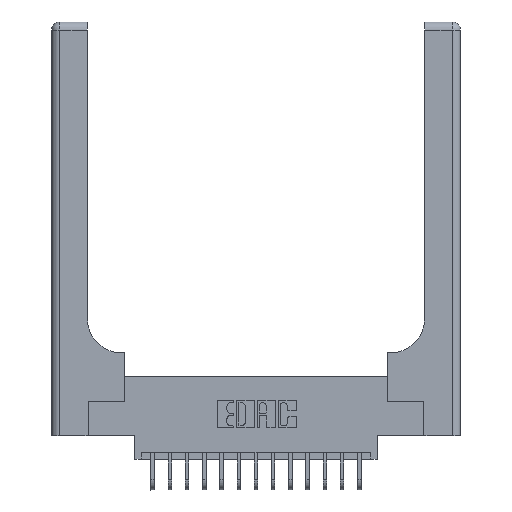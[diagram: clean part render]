
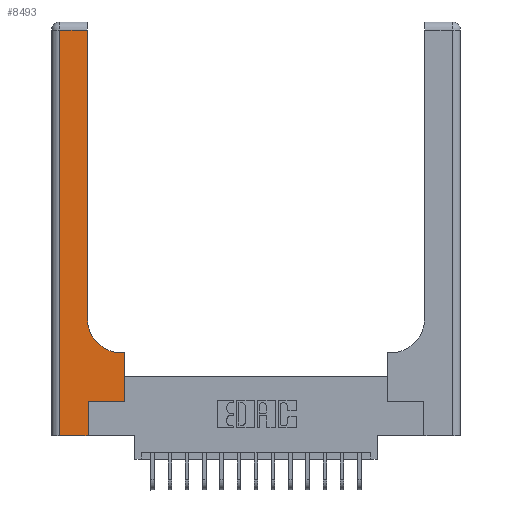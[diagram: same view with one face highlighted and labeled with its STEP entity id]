
A CAD part, top view. The second image highlights one B-rep face of the part: STEP entity #8493.
In plain terms, the highlighted planar face has unit normal (0, 0, 1).
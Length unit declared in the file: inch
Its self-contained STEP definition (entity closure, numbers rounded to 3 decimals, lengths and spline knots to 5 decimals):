
#258 = CARTESIAN_POINT ( 'NONE',  ( 0.26, 0.85, 0.37 ) ) ;
#544 = VERTEX_POINT ( 'NONE', #15797 ) ;
#574 = EDGE_CURVE ( 'NONE', #988, #16833, #8580, .T. ) ;
#685 = CARTESIAN_POINT ( 'NONE',  ( 0.265, 0., 0.37 ) ) ;
#988 = VERTEX_POINT ( 'NONE', #12697 ) ;
#1490 = DIRECTION ( 'NONE',  ( 0., 0., -1. ) ) ;
#1655 = FACE_OUTER_BOUND ( 'NONE', #15881, .T. ) ;
#2187 = VECTOR ( 'NONE', #7124, 39.37008 ) ;
#3043 = CARTESIAN_POINT ( 'NONE',  ( 0.528, 0.6, 0.37 ) ) ;
#3172 = EDGE_CURVE ( 'NONE', #544, #18215, #10111, .T. ) ;
#3312 = VECTOR ( 'NONE', #18444, 39.37008 ) ;
#3699 = DIRECTION ( 'NONE',  ( 0., 1., 0. ) ) ;
#4691 = ORIENTED_EDGE ( 'NONE', *, *, #3172, .T. ) ;
#5363 = EDGE_CURVE ( 'NONE', #16833, #6987, #13559, .T. ) ;
#5413 = VECTOR ( 'NONE', #5875, 39.37008 ) ;
#5875 = DIRECTION ( 'NONE',  ( -1., 0., 0. ) ) ;
#6525 = VERTEX_POINT ( 'NONE', #685 ) ;
#6743 = VECTOR ( 'NONE', #18944, 39.37008 ) ;
#6987 = VERTEX_POINT ( 'NONE', #11197 ) ;
#7124 = DIRECTION ( 'NONE',  ( 0., 1., 0. ) ) ;
#7527 = EDGE_CURVE ( 'NONE', #6525, #14617, #11607, .T. ) ;
#7754 = DIRECTION ( 'NONE',  ( 1., 0., 0. ) ) ;
#7800 = DIRECTION ( 'NONE',  ( -1., 0., 0. ) ) ;
#8045 = EDGE_CURVE ( 'NONE', #18215, #6525, #16307, .T. ) ;
#8174 = ORIENTED_EDGE ( 'NONE', *, *, #14600, .T. ) ;
#8195 = EDGE_CURVE ( 'NONE', #12801, #8676, #13699, .T. ) ;
#8493 = ADVANCED_FACE ( 'NONE', ( #1655 ), #19212, .F. ) ;
#8580 = LINE ( 'NONE', #11336, #2187 ) ;
#8676 = VERTEX_POINT ( 'NONE', #18752 ) ;
#8742 = AXIS2_PLACEMENT_3D ( 'NONE', #18163, #16744, #12337 ) ;
#8985 = CARTESIAN_POINT ( 'NONE',  ( 0., 0., 0.37 ) ) ;
#9067 = CARTESIAN_POINT ( 'NONE',  ( 0.26, 0.6, 0.37 ) ) ;
#9214 = EDGE_CURVE ( 'NONE', #8676, #544, #17437, .T. ) ;
#9702 = VECTOR ( 'NONE', #7754, 39.37008 ) ;
#10111 = LINE ( 'NONE', #10666, #10379 ) ;
#10379 = VECTOR ( 'NONE', #14846, 39.37008 ) ;
#10666 = CARTESIAN_POINT ( 'NONE',  ( 0.06, 3., 0.37 ) ) ;
#10813 = CARTESIAN_POINT ( 'NONE',  ( 0.26, 3., 0.37 ) ) ;
#10923 = VECTOR ( 'NONE', #3699, 39.37008 ) ;
#10976 = AXIS2_PLACEMENT_3D ( 'NONE', #13743, #1490, #7800 ) ;
#11197 = CARTESIAN_POINT ( 'NONE',  ( 0.51, 0.6, 0.37 ) ) ;
#11312 = EDGE_CURVE ( 'NONE', #6987, #12801, #18804, .T. ) ;
#11336 = CARTESIAN_POINT ( 'NONE',  ( 0.528, 0.25, 0.37 ) ) ;
#11607 = LINE ( 'NONE', #18727, #10923 ) ;
#12337 = DIRECTION ( 'NONE',  ( 1., 0., 0. ) ) ;
#12697 = CARTESIAN_POINT ( 'NONE',  ( 0.528, 0.25, 0.37 ) ) ;
#12801 = VERTEX_POINT ( 'NONE', #258 ) ;
#13238 = ORIENTED_EDGE ( 'NONE', *, *, #7527, .T. ) ;
#13462 = ORIENTED_EDGE ( 'NONE', *, *, #9214, .T. ) ;
#13559 = LINE ( 'NONE', #9067, #6743 ) ;
#13699 = LINE ( 'NONE', #10813, #3312 ) ;
#13743 = CARTESIAN_POINT ( 'NONE',  ( 0., 3., 0.37 ) ) ;
#14434 = ORIENTED_EDGE ( 'NONE', *, *, #11312, .T. ) ;
#14600 = EDGE_CURVE ( 'NONE', #14617, #988, #17680, .T. ) ;
#14617 = VERTEX_POINT ( 'NONE', #16838 ) ;
#14788 = CARTESIAN_POINT ( 'NONE',  ( 0.06, 0., 0.37 ) ) ;
#14846 = DIRECTION ( 'NONE',  ( 0., -1., 0. ) ) ;
#15797 = CARTESIAN_POINT ( 'NONE',  ( 0.06, 2.94, 0.37 ) ) ;
#15881 = EDGE_LOOP ( 'NONE', ( #18851, #13462, #4691, #17531, #13238, #8174, #16918, #19408, #14434 ) ) ;
#16222 = CARTESIAN_POINT ( 'NONE',  ( 0., 2.94, 0.37 ) ) ;
#16307 = LINE ( 'NONE', #8985, #9702 ) ;
#16524 = VECTOR ( 'NONE', #18193, 39.37008 ) ;
#16635 = CARTESIAN_POINT ( 'NONE',  ( 0.265, 0.25, 0.37 ) ) ;
#16744 = DIRECTION ( 'NONE',  ( 0., 0., -1. ) ) ;
#16833 = VERTEX_POINT ( 'NONE', #3043 ) ;
#16838 = CARTESIAN_POINT ( 'NONE',  ( 0.265, 0.25, 0.37 ) ) ;
#16918 = ORIENTED_EDGE ( 'NONE', *, *, #574, .T. ) ;
#17437 = LINE ( 'NONE', #16222, #5413 ) ;
#17531 = ORIENTED_EDGE ( 'NONE', *, *, #8045, .T. ) ;
#17680 = LINE ( 'NONE', #16635, #16524 ) ;
#18163 = CARTESIAN_POINT ( 'NONE',  ( 0.51, 0.85, 0.37 ) ) ;
#18193 = DIRECTION ( 'NONE',  ( 1., 0., 0. ) ) ;
#18215 = VERTEX_POINT ( 'NONE', #14788 ) ;
#18444 = DIRECTION ( 'NONE',  ( 0., 1., 0. ) ) ;
#18727 = CARTESIAN_POINT ( 'NONE',  ( 0.265, 0., 0.37 ) ) ;
#18752 = CARTESIAN_POINT ( 'NONE',  ( 0.26, 2.94, 0.37 ) ) ;
#18804 = CIRCLE ( 'NONE', #8742, 0.25 ) ;
#18851 = ORIENTED_EDGE ( 'NONE', *, *, #8195, .T. ) ;
#18944 = DIRECTION ( 'NONE',  ( -1., 0., 0. ) ) ;
#19212 = PLANE ( 'NONE',  #10976 ) ;
#19408 = ORIENTED_EDGE ( 'NONE', *, *, #5363, .T. ) ;
